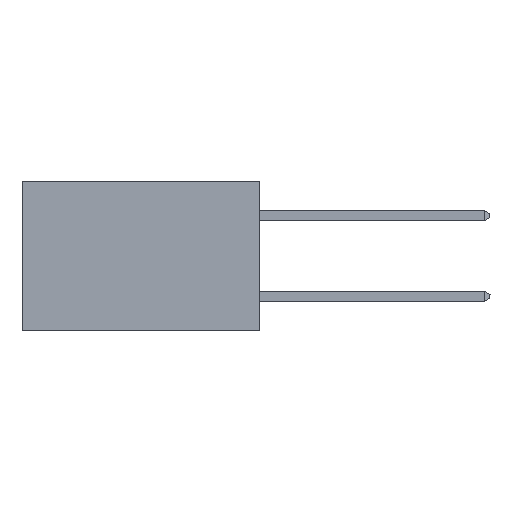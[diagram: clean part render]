
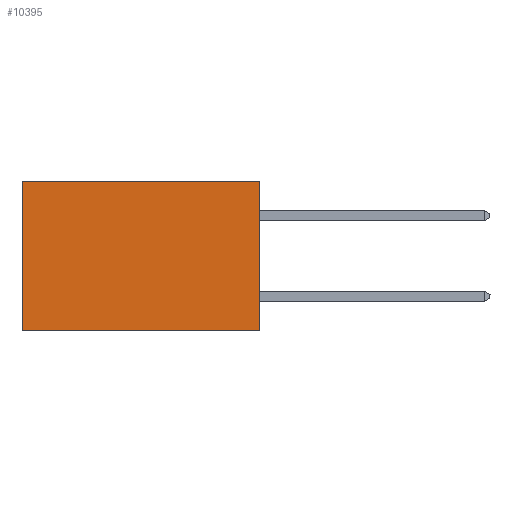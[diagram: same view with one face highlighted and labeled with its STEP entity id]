
A CAD part, left-side view. The second image highlights one B-rep face of the part: STEP entity #10395.
In plain terms, the highlighted planar face has unit normal (-1, 0, 0).
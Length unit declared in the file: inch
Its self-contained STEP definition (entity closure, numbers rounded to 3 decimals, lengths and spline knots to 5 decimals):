
#53 = CARTESIAN_POINT ( 'NONE',  ( 0.277, 0., -0.37 ) ) ;
#116 = LINE ( 'NONE', #1815, #4578 ) ;
#240 = ORIENTED_EDGE ( 'NONE', *, *, #4435, .T. ) ;
#856 = DIRECTION ( 'NONE',  ( 0., 0., -1. ) ) ;
#1042 = VERTEX_POINT ( 'NONE', #9730 ) ;
#1209 = LINE ( 'NONE', #3663, #7904 ) ;
#1535 = VERTEX_POINT ( 'NONE', #9628 ) ;
#1605 = CARTESIAN_POINT ( 'NONE',  ( 0.277, 0.59, -0.37 ) ) ;
#1797 = DIRECTION ( 'NONE',  ( 0., 1., 0. ) ) ;
#1815 = CARTESIAN_POINT ( 'NONE',  ( 0.277, 0., -0.37 ) ) ;
#3663 = CARTESIAN_POINT ( 'NONE',  ( 0.277, 0., -0.37 ) ) ;
#3901 = ORIENTED_EDGE ( 'NONE', *, *, #10964, .T. ) ;
#3993 = VECTOR ( 'NONE', #4125, 39.37008 ) ;
#4125 = DIRECTION ( 'NONE',  ( 0., 1., 0. ) ) ;
#4149 = ORIENTED_EDGE ( 'NONE', *, *, #8330, .F. ) ;
#4435 = EDGE_CURVE ( 'NONE', #10351, #1042, #8309, .T. ) ;
#4578 = VECTOR ( 'NONE', #1797, 39.37008 ) ;
#4702 = VERTEX_POINT ( 'NONE', #53 ) ;
#4717 = EDGE_CURVE ( 'NONE', #10351, #4702, #1209, .T. ) ;
#4871 = FACE_OUTER_BOUND ( 'NONE', #7137, .T. ) ;
#5010 = CARTESIAN_POINT ( 'NONE',  ( 0.277, 0., 0. ) ) ;
#5266 = PLANE ( 'NONE',  #9296 ) ;
#5581 = VECTOR ( 'NONE', #8544, 39.37008 ) ;
#6144 = DIRECTION ( 'NONE',  ( 1., 0., 0. ) ) ;
#6731 = ORIENTED_EDGE ( 'NONE', *, *, #4717, .F. ) ;
#7137 = EDGE_LOOP ( 'NONE', ( #3901, #4149, #6731, #240 ) ) ;
#7586 = CARTESIAN_POINT ( 'NONE',  ( 0.277, 0., 0. ) ) ;
#7904 = VECTOR ( 'NONE', #10463, 39.37008 ) ;
#8309 = LINE ( 'NONE', #5010, #3993 ) ;
#8330 = EDGE_CURVE ( 'NONE', #4702, #1535, #116, .T. ) ;
#8544 = DIRECTION ( 'NONE',  ( 0., 0., -1. ) ) ;
#9296 = AXIS2_PLACEMENT_3D ( 'NONE', #11176, #6144, #856 ) ;
#9628 = CARTESIAN_POINT ( 'NONE',  ( 0.277, 0.59, -0.37 ) ) ;
#9730 = CARTESIAN_POINT ( 'NONE',  ( 0.277, 0.59, 0. ) ) ;
#10318 = LINE ( 'NONE', #1605, #5581 ) ;
#10351 = VERTEX_POINT ( 'NONE', #7586 ) ;
#10395 = ADVANCED_FACE ( 'NONE', ( #4871 ), #5266, .F. ) ;
#10463 = DIRECTION ( 'NONE',  ( 0., 0., -1. ) ) ;
#10964 = EDGE_CURVE ( 'NONE', #1042, #1535, #10318, .T. ) ;
#11176 = CARTESIAN_POINT ( 'NONE',  ( 0.277, 0., -0.37 ) ) ;
